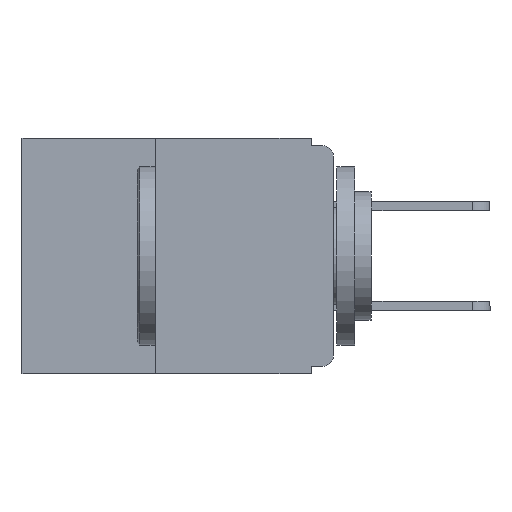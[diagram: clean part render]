
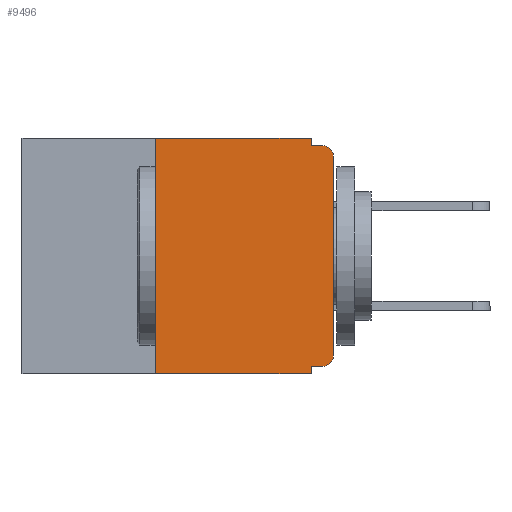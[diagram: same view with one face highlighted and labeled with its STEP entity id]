
A CAD part, left-side view. The second image highlights one B-rep face of the part: STEP entity #9496.
In plain terms, the highlighted planar face has unit normal (-1, 0, 0).
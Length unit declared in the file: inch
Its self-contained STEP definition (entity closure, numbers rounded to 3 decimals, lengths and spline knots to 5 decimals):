
#99 = CARTESIAN_POINT ( 'NONE',  ( 0., 0., 0. ) ) ;
#418 = DIRECTION ( 'NONE',  ( 0., 0., -1. ) ) ;
#472 = CARTESIAN_POINT ( 'NONE',  ( 0., 0.437, -0.33 ) ) ;
#713 = ORIENTED_EDGE ( 'NONE', *, *, #13651, .T. ) ;
#979 = DIRECTION ( 'NONE',  ( 0., -1., 0. ) ) ;
#1247 = DIRECTION ( 'NONE',  ( 0., 0., 1. ) ) ;
#1516 = DIRECTION ( 'NONE',  ( 0., 0., 1. ) ) ;
#1704 = VECTOR ( 'NONE', #3431, 39.37008 ) ;
#1965 = VECTOR ( 'NONE', #10731, 39.37008 ) ;
#2217 = LINE ( 'NONE', #11757, #7793 ) ;
#2535 = ORIENTED_EDGE ( 'NONE', *, *, #10645, .F. ) ;
#2662 = LINE ( 'NONE', #472, #11842 ) ;
#3032 = CARTESIAN_POINT ( 'NONE',  ( 0., 0., -0.025 ) ) ;
#3313 = LINE ( 'NONE', #13713, #13266 ) ;
#3431 = DIRECTION ( 'NONE',  ( 0., -1., 0. ) ) ;
#3542 = VECTOR ( 'NONE', #1247, 39.37008 ) ;
#3558 = DIRECTION ( 'NONE',  ( 1., 0., 0. ) ) ;
#3945 = DIRECTION ( 'NONE',  ( 0., -1., 0. ) ) ;
#3986 = DIRECTION ( 'NONE',  ( -1., 0., 0. ) ) ;
#4234 = EDGE_CURVE ( 'NONE', #13200, #6679, #14381, .T. ) ;
#4455 = CARTESIAN_POINT ( 'NONE',  ( 0., 0., -0.01 ) ) ;
#4914 = CARTESIAN_POINT ( 'NONE',  ( 0., 0.031, -0.32 ) ) ;
#5872 = EDGE_CURVE ( 'NONE', #11940, #13130, #2217, .T. ) ;
#6679 = VERTEX_POINT ( 'NONE', #13083 ) ;
#6694 = CARTESIAN_POINT ( 'NONE',  ( 0., 0., -0.305 ) ) ;
#7050 = VERTEX_POINT ( 'NONE', #9868 ) ;
#7060 = CIRCLE ( 'NONE', #7754, 0.015 ) ;
#7475 = DIRECTION ( 'NONE',  ( -1., 0., 0. ) ) ;
#7754 = AXIS2_PLACEMENT_3D ( 'NONE', #11167, #3986, #12401 ) ;
#7793 = VECTOR ( 'NONE', #8407, 39.37008 ) ;
#7849 = CARTESIAN_POINT ( 'NONE',  ( 0., 0.031, -0.33 ) ) ;
#8328 = ORIENTED_EDGE ( 'NONE', *, *, #4234, .F. ) ;
#8407 = DIRECTION ( 'NONE',  ( 0., 1., 0. ) ) ;
#8409 = CARTESIAN_POINT ( 'NONE',  ( 0., 0.015, -0.32 ) ) ;
#8510 = CARTESIAN_POINT ( 'NONE',  ( 0., 0.031, 0. ) ) ;
#8539 = CARTESIAN_POINT ( 'NONE',  ( 0., 0.25, -0.33 ) ) ;
#8560 = VERTEX_POINT ( 'NONE', #3032 ) ;
#8636 = EDGE_LOOP ( 'NONE', ( #713, #13395, #11326, #2535, #10006, #8328, #8705, #12677, #10960, #11338 ) ) ;
#8705 = ORIENTED_EDGE ( 'NONE', *, *, #12605, .T. ) ;
#8778 = VECTOR ( 'NONE', #979, 39.37008 ) ;
#9025 = EDGE_CURVE ( 'NONE', #11940, #13453, #12121, .T. ) ;
#9151 = LINE ( 'NONE', #4455, #8778 ) ;
#9496 = ADVANCED_FACE ( 'NONE', ( #14833 ), #11903, .F. ) ;
#9868 = CARTESIAN_POINT ( 'NONE',  ( 0., 0.015, -0.01 ) ) ;
#10006 = ORIENTED_EDGE ( 'NONE', *, *, #14215, .F. ) ;
#10587 = CARTESIAN_POINT ( 'NONE',  ( 0., 0.437, 0. ) ) ;
#10645 = EDGE_CURVE ( 'NONE', #13885, #10794, #14264, .T. ) ;
#10706 = CARTESIAN_POINT ( 'NONE',  ( 0., 0.437, 0. ) ) ;
#10731 = DIRECTION ( 'NONE',  ( 0., 0., -1. ) ) ;
#10794 = VERTEX_POINT ( 'NONE', #12192 ) ;
#10960 = ORIENTED_EDGE ( 'NONE', *, *, #5872, .F. ) ;
#11167 = CARTESIAN_POINT ( 'NONE',  ( 0., 0.015, -0.025 ) ) ;
#11213 = LINE ( 'NONE', #10587, #1704 ) ;
#11235 = VECTOR ( 'NONE', #1516, 39.37008 ) ;
#11326 = ORIENTED_EDGE ( 'NONE', *, *, #14155, .F. ) ;
#11338 = ORIENTED_EDGE ( 'NONE', *, *, #9025, .T. ) ;
#11757 = CARTESIAN_POINT ( 'NONE',  ( 0., 0., -0.32 ) ) ;
#11842 = VECTOR ( 'NONE', #3945, 39.37008 ) ;
#11903 = PLANE ( 'NONE',  #12362 ) ;
#11940 = VERTEX_POINT ( 'NONE', #8409 ) ;
#11962 = DIRECTION ( 'NONE',  ( 0., 0., -1. ) ) ;
#12121 = CIRCLE ( 'NONE', #13043, 0.015 ) ;
#12192 = CARTESIAN_POINT ( 'NONE',  ( 0., 0.031, -0.01 ) ) ;
#12362 = AXIS2_PLACEMENT_3D ( 'NONE', #10706, #3558, #11962 ) ;
#12401 = DIRECTION ( 'NONE',  ( 0., 0., -1. ) ) ;
#12605 = EDGE_CURVE ( 'NONE', #13200, #14678, #2662, .T. ) ;
#12677 = ORIENTED_EDGE ( 'NONE', *, *, #15169, .F. ) ;
#13043 = AXIS2_PLACEMENT_3D ( 'NONE', #14636, #7475, #418 ) ;
#13083 = CARTESIAN_POINT ( 'NONE',  ( 0., 0.25, 0. ) ) ;
#13130 = VERTEX_POINT ( 'NONE', #4914 ) ;
#13137 = LINE ( 'NONE', #99, #3542 ) ;
#13145 = CARTESIAN_POINT ( 'NONE',  ( 0., 0.031, 0. ) ) ;
#13200 = VERTEX_POINT ( 'NONE', #8539 ) ;
#13266 = VECTOR ( 'NONE', #14855, 39.37008 ) ;
#13395 = ORIENTED_EDGE ( 'NONE', *, *, #14504, .T. ) ;
#13453 = VERTEX_POINT ( 'NONE', #6694 ) ;
#13651 = EDGE_CURVE ( 'NONE', #13453, #8560, #13137, .T. ) ;
#13713 = CARTESIAN_POINT ( 'NONE',  ( 0., 0.031, -0.33 ) ) ;
#13885 = VERTEX_POINT ( 'NONE', #8510 ) ;
#14155 = EDGE_CURVE ( 'NONE', #10794, #7050, #9151, .T. ) ;
#14215 = EDGE_CURVE ( 'NONE', #6679, #13885, #11213, .T. ) ;
#14264 = LINE ( 'NONE', #13145, #1965 ) ;
#14381 = LINE ( 'NONE', #14466, #11235 ) ;
#14466 = CARTESIAN_POINT ( 'NONE',  ( 0., 0.25, -0.33 ) ) ;
#14504 = EDGE_CURVE ( 'NONE', #8560, #7050, #7060, .T. ) ;
#14636 = CARTESIAN_POINT ( 'NONE',  ( 0., 0.015, -0.305 ) ) ;
#14678 = VERTEX_POINT ( 'NONE', #7849 ) ;
#14833 = FACE_OUTER_BOUND ( 'NONE', #8636, .T. ) ;
#14855 = DIRECTION ( 'NONE',  ( 0., 0., -1. ) ) ;
#15169 = EDGE_CURVE ( 'NONE', #13130, #14678, #3313, .T. ) ;
